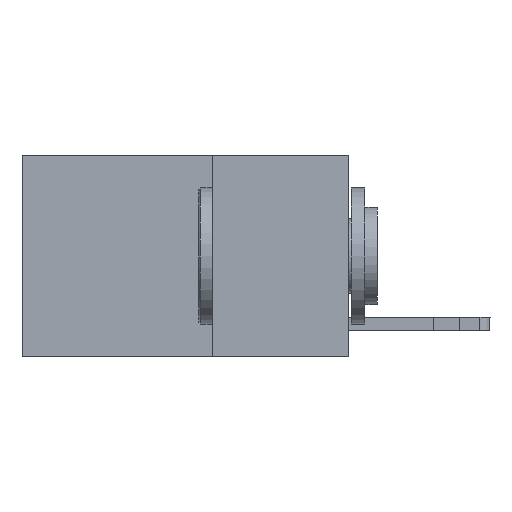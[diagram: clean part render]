
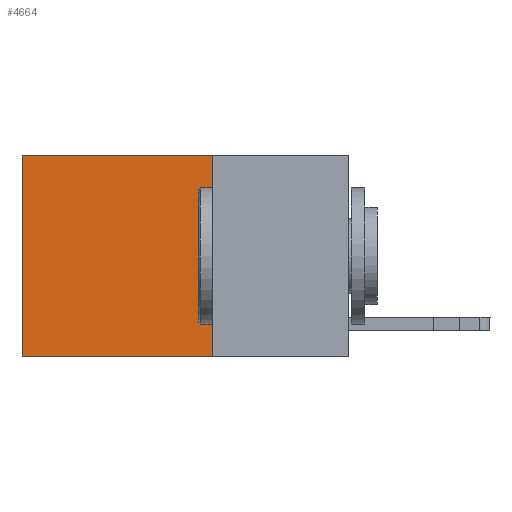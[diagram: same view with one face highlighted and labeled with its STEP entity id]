
A CAD part, left-side view. The second image highlights one B-rep face of the part: STEP entity #4664.
In plain terms, the highlighted planar face has unit normal (-1, 0, 0).
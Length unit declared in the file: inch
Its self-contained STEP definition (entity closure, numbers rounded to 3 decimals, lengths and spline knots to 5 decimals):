
#10 = DIRECTION ( 'NONE',  ( 1., 0., 0. ) ) ;
#536 = DIRECTION ( 'NONE',  ( 0., 1., 0. ) ) ;
#958 = CARTESIAN_POINT ( 'NONE',  ( 0.2625, 0.6, -0.37 ) ) ;
#1025 = EDGE_CURVE ( 'NONE', #1757, #20146, #12710, .T. ) ;
#1180 = DIRECTION ( 'NONE',  ( 0., 0., -1. ) ) ;
#1268 = CARTESIAN_POINT ( 'NONE',  ( 0.2625, 0.6, 0. ) ) ;
#1757 = VERTEX_POINT ( 'NONE', #2487 ) ;
#2040 = CARTESIAN_POINT ( 'NONE',  ( 0.2625, 0.25, 0. ) ) ;
#2487 = CARTESIAN_POINT ( 'NONE',  ( 0.2625, 0.25, 0. ) ) ;
#2580 = ORIENTED_EDGE ( 'NONE', *, *, #16158, .F. ) ;
#3240 = CARTESIAN_POINT ( 'NONE',  ( 0.2625, 0.25, -0.37 ) ) ;
#3300 = CARTESIAN_POINT ( 'NONE',  ( 0.2625, 0.25, -0.37 ) ) ;
#3308 = VECTOR ( 'NONE', #536, 39.37008 ) ;
#3807 = EDGE_CURVE ( 'NONE', #20146, #16427, #18603, .T. ) ;
#4201 = EDGE_LOOP ( 'NONE', ( #20999, #17338, #2580, #6792 ) ) ;
#4580 = EDGE_CURVE ( 'NONE', #20872, #16427, #20528, .T. ) ;
#4664 = ADVANCED_FACE ( 'NONE', ( #18887 ), #14029, .F. ) ;
#5044 = DIRECTION ( 'NONE',  ( 0., 1., 0. ) ) ;
#5069 = VECTOR ( 'NONE', #1180, 39.37008 ) ;
#5324 = VECTOR ( 'NONE', #14384, 39.37008 ) ;
#6511 = VECTOR ( 'NONE', #5044, 39.37008 ) ;
#6792 = ORIENTED_EDGE ( 'NONE', *, *, #1025, .T. ) ;
#7523 = CARTESIAN_POINT ( 'NONE',  ( 0.2625, 0.25, 0. ) ) ;
#9493 = LINE ( 'NONE', #2040, #5324 ) ;
#10560 = CARTESIAN_POINT ( 'NONE',  ( 0.2625, 0.25, 0. ) ) ;
#11672 = AXIS2_PLACEMENT_3D ( 'NONE', #10560, #10, #12333 ) ;
#12333 = DIRECTION ( 'NONE',  ( 0., 0., -1. ) ) ;
#12710 = LINE ( 'NONE', #7523, #3308 ) ;
#13546 = CARTESIAN_POINT ( 'NONE',  ( 0.2625, 0.6, 0. ) ) ;
#14029 = PLANE ( 'NONE',  #11672 ) ;
#14384 = DIRECTION ( 'NONE',  ( 0., 0., -1. ) ) ;
#16158 = EDGE_CURVE ( 'NONE', #1757, #20872, #9493, .T. ) ;
#16427 = VERTEX_POINT ( 'NONE', #958 ) ;
#17338 = ORIENTED_EDGE ( 'NONE', *, *, #4580, .F. ) ;
#18603 = LINE ( 'NONE', #13546, #5069 ) ;
#18887 = FACE_OUTER_BOUND ( 'NONE', #4201, .T. ) ;
#20146 = VERTEX_POINT ( 'NONE', #1268 ) ;
#20528 = LINE ( 'NONE', #3300, #6511 ) ;
#20872 = VERTEX_POINT ( 'NONE', #3240 ) ;
#20999 = ORIENTED_EDGE ( 'NONE', *, *, #3807, .T. ) ;
